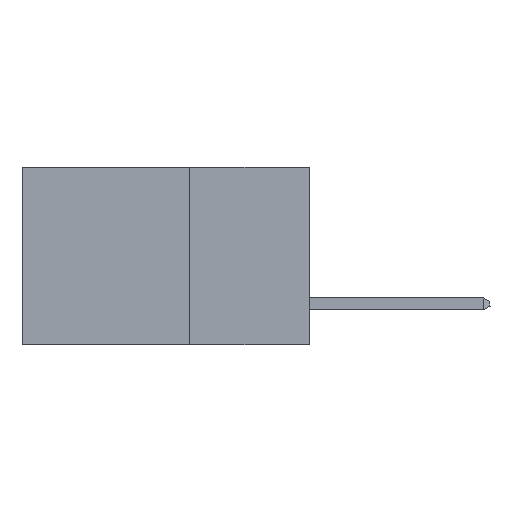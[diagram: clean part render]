
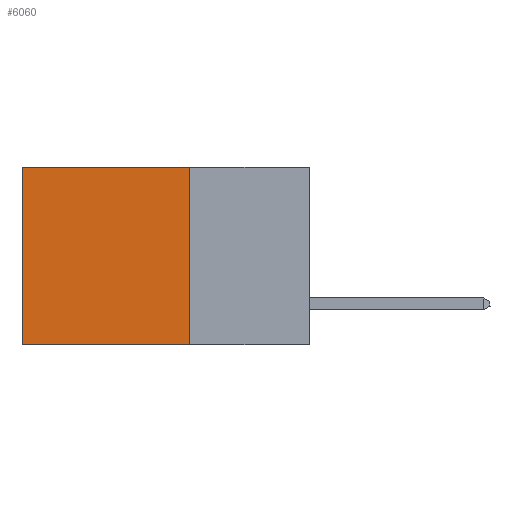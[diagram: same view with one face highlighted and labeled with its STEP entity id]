
A CAD part, left-side view. The second image highlights one B-rep face of the part: STEP entity #6060.
In plain terms, the highlighted planar face has unit normal (-1, 0, 0).
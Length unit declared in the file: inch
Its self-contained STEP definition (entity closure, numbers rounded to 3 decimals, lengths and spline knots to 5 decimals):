
#205 = EDGE_CURVE ( 'NONE', #419, #27264, #31953, .T. ) ;
#419 = VERTEX_POINT ( 'NONE', #17688 ) ;
#634 = VECTOR ( 'NONE', #43464, 39.37008 ) ;
#3333 = EDGE_CURVE ( 'NONE', #19116, #5194, #11644, .T. ) ;
#5194 = VERTEX_POINT ( 'NONE', #33050 ) ;
#6060 = ADVANCED_FACE ( 'NONE', ( #42730 ), #44897, .F. ) ;
#6278 = DIRECTION ( 'NONE',  ( 0., 1., 0. ) ) ;
#7923 = CARTESIAN_POINT ( 'NONE',  ( 0.2875, 0.6, 0. ) ) ;
#9885 = CARTESIAN_POINT ( 'NONE',  ( 0.2875, 0.25, -0.37 ) ) ;
#11212 = CARTESIAN_POINT ( 'NONE',  ( 0.2875, 0.25, -0.37 ) ) ;
#11644 = LINE ( 'NONE', #9885, #44103 ) ;
#12627 = ORIENTED_EDGE ( 'NONE', *, *, #30890, .T. ) ;
#13357 = ORIENTED_EDGE ( 'NONE', *, *, #3333, .F. ) ;
#17688 = CARTESIAN_POINT ( 'NONE',  ( 0.2875, 0.25, 0. ) ) ;
#19113 = EDGE_LOOP ( 'NONE', ( #12627, #13357, #29440, #28313 ) ) ;
#19116 = VERTEX_POINT ( 'NONE', #11212 ) ;
#21182 = LINE ( 'NONE', #31438, #39087 ) ;
#21288 = DIRECTION ( 'NONE',  ( 0., 1., 0. ) ) ;
#22430 = VECTOR ( 'NONE', #21288, 39.37008 ) ;
#25351 = LINE ( 'NONE', #29697, #634 ) ;
#27264 = VERTEX_POINT ( 'NONE', #7923 ) ;
#28163 = AXIS2_PLACEMENT_3D ( 'NONE', #37496, #45207, #37651 ) ;
#28313 = ORIENTED_EDGE ( 'NONE', *, *, #205, .T. ) ;
#28463 = DIRECTION ( 'NONE',  ( 0., 0., -1. ) ) ;
#29440 = ORIENTED_EDGE ( 'NONE', *, *, #44360, .F. ) ;
#29697 = CARTESIAN_POINT ( 'NONE',  ( 0.2875, 0.25, 0. ) ) ;
#30890 = EDGE_CURVE ( 'NONE', #27264, #5194, #21182, .T. ) ;
#31438 = CARTESIAN_POINT ( 'NONE',  ( 0.2875, 0.6, 0. ) ) ;
#31650 = CARTESIAN_POINT ( 'NONE',  ( 0.2875, 0.25, 0. ) ) ;
#31953 = LINE ( 'NONE', #31650, #22430 ) ;
#33050 = CARTESIAN_POINT ( 'NONE',  ( 0.2875, 0.6, -0.37 ) ) ;
#37496 = CARTESIAN_POINT ( 'NONE',  ( 0.2875, 0.25, 0. ) ) ;
#37651 = DIRECTION ( 'NONE',  ( 0., 0., -1. ) ) ;
#39087 = VECTOR ( 'NONE', #28463, 39.37008 ) ;
#42730 = FACE_OUTER_BOUND ( 'NONE', #19113, .T. ) ;
#43464 = DIRECTION ( 'NONE',  ( 0., 0., -1. ) ) ;
#44103 = VECTOR ( 'NONE', #6278, 39.37008 ) ;
#44360 = EDGE_CURVE ( 'NONE', #419, #19116, #25351, .T. ) ;
#44897 = PLANE ( 'NONE',  #28163 ) ;
#45207 = DIRECTION ( 'NONE',  ( 1., 0., 0. ) ) ;
